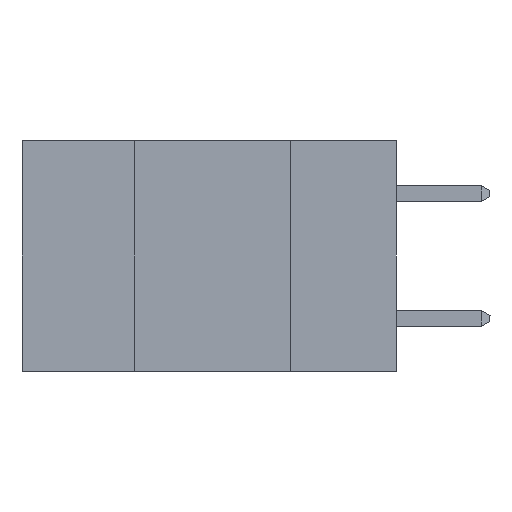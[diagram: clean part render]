
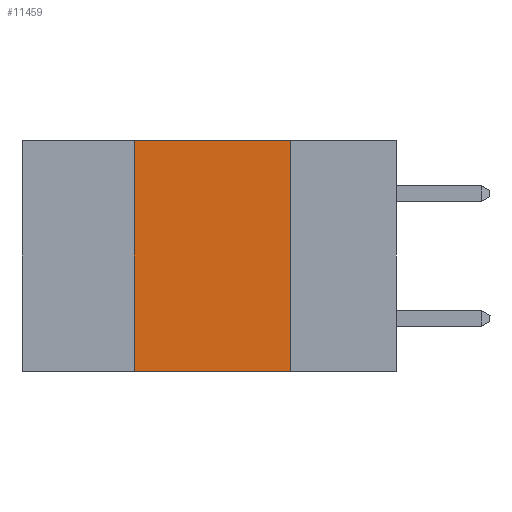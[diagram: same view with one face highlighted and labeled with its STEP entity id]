
A CAD part, left-side view. The second image highlights one B-rep face of the part: STEP entity #11459.
In plain terms, the highlighted planar face has unit normal (-1, 0, 0).
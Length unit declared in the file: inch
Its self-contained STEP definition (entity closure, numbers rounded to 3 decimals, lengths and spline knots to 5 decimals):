
#213 = DIRECTION ( 'NONE',  ( 0., -1., 0. ) ) ;
#1540 = CARTESIAN_POINT ( 'NONE',  ( 0., 0.6, 0. ) ) ;
#1708 = VECTOR ( 'NONE', #12448, 39.37008 ) ;
#1783 = EDGE_CURVE ( 'NONE', #12360, #6270, #12793, .T. ) ;
#2045 = CARTESIAN_POINT ( 'NONE',  ( 0., 0.6, 0. ) ) ;
#2387 = VERTEX_POINT ( 'NONE', #10373 ) ;
#2484 = VECTOR ( 'NONE', #10576, 39.37008 ) ;
#3054 = DIRECTION ( 'NONE',  ( 0., 0., -1. ) ) ;
#4358 = LINE ( 'NONE', #7436, #1708 ) ;
#4527 = EDGE_CURVE ( 'NONE', #6270, #8648, #4358, .T. ) ;
#4656 = CARTESIAN_POINT ( 'NONE',  ( 0., 0.6, -0.37 ) ) ;
#4758 = DIRECTION ( 'NONE',  ( 0., 0., 1. ) ) ;
#6144 = AXIS2_PLACEMENT_3D ( 'NONE', #2045, #9009, #3054 ) ;
#6238 = ORIENTED_EDGE ( 'NONE', *, *, #1783, .F. ) ;
#6270 = VERTEX_POINT ( 'NONE', #8308 ) ;
#6542 = ORIENTED_EDGE ( 'NONE', *, *, #8583, .T. ) ;
#6764 = EDGE_LOOP ( 'NONE', ( #11239, #6238, #11565, #6542 ) ) ;
#7073 = LINE ( 'NONE', #8683, #7402 ) ;
#7087 = FACE_OUTER_BOUND ( 'NONE', #6764, .T. ) ;
#7402 = VECTOR ( 'NONE', #4758, 39.37008 ) ;
#7436 = CARTESIAN_POINT ( 'NONE',  ( 0., 0.17, -0.37 ) ) ;
#7499 = VECTOR ( 'NONE', #213, 39.37008 ) ;
#8005 = PLANE ( 'NONE',  #6144 ) ;
#8308 = CARTESIAN_POINT ( 'NONE',  ( 0., 0.17, 0. ) ) ;
#8583 = EDGE_CURVE ( 'NONE', #2387, #8648, #10421, .T. ) ;
#8648 = VERTEX_POINT ( 'NONE', #11740 ) ;
#8683 = CARTESIAN_POINT ( 'NONE',  ( 0., 0.42, -0.37 ) ) ;
#9009 = DIRECTION ( 'NONE',  ( 1., 0., 0. ) ) ;
#10373 = CARTESIAN_POINT ( 'NONE',  ( 0., 0.42, -0.37 ) ) ;
#10421 = LINE ( 'NONE', #4656, #2484 ) ;
#10576 = DIRECTION ( 'NONE',  ( 0., -1., 0. ) ) ;
#11239 = ORIENTED_EDGE ( 'NONE', *, *, #4527, .F. ) ;
#11459 = ADVANCED_FACE ( 'NONE', ( #7087 ), #8005, .F. ) ;
#11565 = ORIENTED_EDGE ( 'NONE', *, *, #11960, .F. ) ;
#11740 = CARTESIAN_POINT ( 'NONE',  ( 0., 0.17, -0.37 ) ) ;
#11960 = EDGE_CURVE ( 'NONE', #2387, #12360, #7073, .T. ) ;
#12342 = CARTESIAN_POINT ( 'NONE',  ( 0., 0.42, 0. ) ) ;
#12360 = VERTEX_POINT ( 'NONE', #12342 ) ;
#12448 = DIRECTION ( 'NONE',  ( 0., 0., -1. ) ) ;
#12793 = LINE ( 'NONE', #1540, #7499 ) ;
